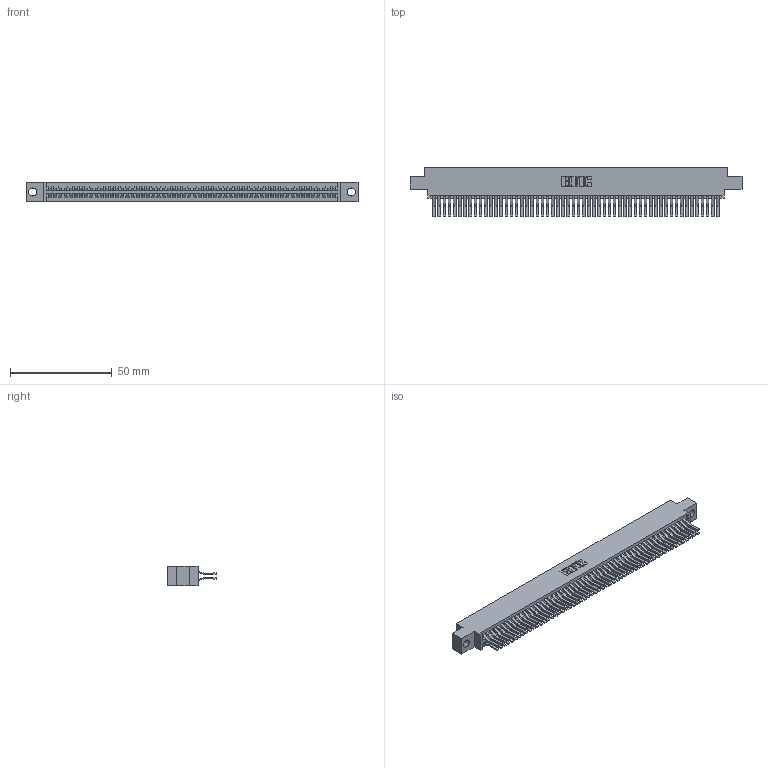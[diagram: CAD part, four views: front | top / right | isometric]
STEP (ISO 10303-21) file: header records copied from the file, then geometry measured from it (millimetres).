
FILE_DESCRIPTION (( 'STEP AP203' ), '1' );
FILE_NAME ('345-112-560-804.STEP', '2018-10-07T17:59:46', ( '' ), ( '' ), 'SwSTEP 2.0', 'SolidWorks 2016', '' );
FILE_SCHEMA (( 'CONFIG_CONTROL_DESIGN' ));
Length unit declared in the file: inch
Products named in the file (3): 345 Part_0.170 Offset - 0.156 Dia-TH; 345-292-001_560 Tail; 345-112-560-804
Assembly tree (113 placements, depth 2):
  345-112-560-804
    345 Part_0.170 Offset - 0.156 Dia-TH
    345-292-001_560 Tail  x112
Bounding box: 163.45 x 24.45 x 9.4 mm (x, y, z)
Volume: 16540.4 mm3; surface area: 26567.4 mm2
Topology: 113 solids, 113 shells, 5954 faces, 17713 edges, 11658 vertices
Faces by surface type: plane 3780, cylinder 2174
Entity records: 42277 total; most frequent: CARTESIAN_POINT 7076, ORIENTED_EDGE 7010, DIRECTION 6225, EDGE_CURVE 3505, LINE 3145, VECTOR 3145, VERTEX_POINT 2334, AXIS2_PLACEMENT_3D 1540
